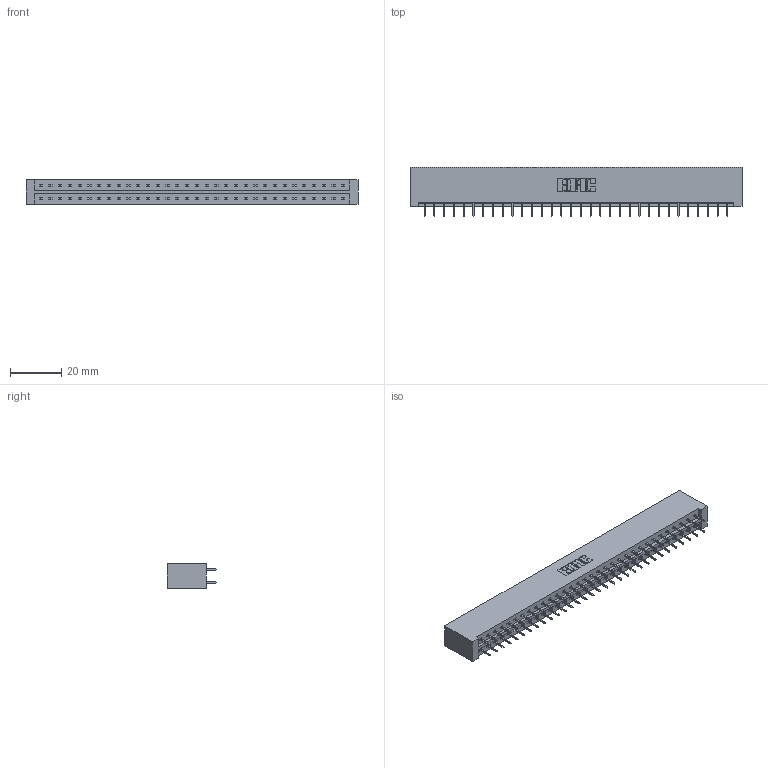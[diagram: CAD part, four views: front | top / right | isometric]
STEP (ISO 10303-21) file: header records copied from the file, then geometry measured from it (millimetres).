
FILE_DESCRIPTION (( 'STEP AP203' ), '1' );
FILE_NAME ('379-064-524-201.STEP', '2020-02-26T18:34:38', ( '' ), ( '' ), 'SwSTEP 2.0', 'SolidWorks 2016', '' );
FILE_SCHEMA (( 'CONFIG_CONTROL_DESIGN' ));
Length unit declared in the file: inch
Products named in the file (3): 345-292-001_345-293-124; 379 Part_Lugless; 379-064-524-201
Assembly tree (65 placements, depth 2):
  379-064-524-201
    379 Part_Lugless
    345-292-001_345-293-124  x64
Bounding box: 129.54 x 19.35 x 9.53 mm (x, y, z)
Volume: 14323.1 mm3; surface area: 15736 mm2
Topology: 65 solids, 65 shells, 3690 faces, 10463 edges, 6718 vertices
Faces by surface type: plane 2754, cylinder 936
Entity records: 21677 total; most frequent: CARTESIAN_POINT 3602, ORIENTED_EDGE 3538, DIRECTION 3089, EDGE_CURVE 1769, VECTOR 1653, LINE 1653, VERTEX_POINT 1174, AXIS2_PLACEMENT_3D 718
